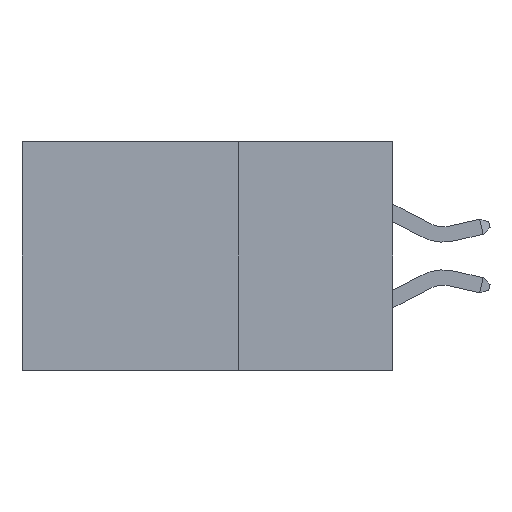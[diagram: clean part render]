
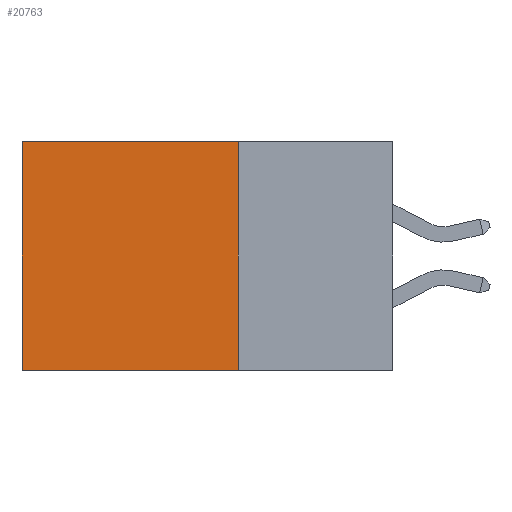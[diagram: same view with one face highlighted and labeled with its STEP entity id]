
A CAD part, left-side view. The second image highlights one B-rep face of the part: STEP entity #20763.
In plain terms, the highlighted planar face has unit normal (-1, 0, 0).
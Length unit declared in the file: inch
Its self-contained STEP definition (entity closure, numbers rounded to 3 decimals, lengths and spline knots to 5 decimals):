
#426 = ORIENTED_EDGE ( 'NONE', *, *, #22774, .F. ) ;
#922 = VERTEX_POINT ( 'NONE', #23130 ) ;
#1095 = VECTOR ( 'NONE', #3715, 39.37008 ) ;
#1285 = VERTEX_POINT ( 'NONE', #10733 ) ;
#1451 = CARTESIAN_POINT ( 'NONE',  ( 0.2875, 0.25, 0. ) ) ;
#2188 = LINE ( 'NONE', #1451, #15929 ) ;
#3715 = DIRECTION ( 'NONE',  ( 0., 0., -1. ) ) ;
#4207 = DIRECTION ( 'NONE',  ( 0., 1., 0. ) ) ;
#5421 = FACE_OUTER_BOUND ( 'NONE', #21174, .T. ) ;
#6524 = LINE ( 'NONE', #10016, #12983 ) ;
#6859 = VERTEX_POINT ( 'NONE', #26353 ) ;
#7999 = AXIS2_PLACEMENT_3D ( 'NONE', #14714, #33502, #17444 ) ;
#10016 = CARTESIAN_POINT ( 'NONE',  ( 0.2875, 0.25, -0.37 ) ) ;
#10733 = CARTESIAN_POINT ( 'NONE',  ( 0.2875, 0.6, -0.37 ) ) ;
#12983 = VECTOR ( 'NONE', #23531, 39.37008 ) ;
#14714 = CARTESIAN_POINT ( 'NONE',  ( 0.2875, 0.25, 0. ) ) ;
#15024 = EDGE_CURVE ( 'NONE', #6859, #922, #34993, .T. ) ;
#15929 = VECTOR ( 'NONE', #4207, 39.37008 ) ;
#16558 = LINE ( 'NONE', #30798, #1095 ) ;
#17122 = VERTEX_POINT ( 'NONE', #29654 ) ;
#17137 = ORIENTED_EDGE ( 'NONE', *, *, #27970, .T. ) ;
#17444 = DIRECTION ( 'NONE',  ( 0., 0., -1. ) ) ;
#19570 = ORIENTED_EDGE ( 'NONE', *, *, #25961, .T. ) ;
#20763 = ADVANCED_FACE ( 'NONE', ( #5421 ), #22733, .F. ) ;
#21174 = EDGE_LOOP ( 'NONE', ( #19570, #426, #25136, #17137 ) ) ;
#22733 = PLANE ( 'NONE',  #7999 ) ;
#22774 = EDGE_CURVE ( 'NONE', #922, #1285, #6524, .T. ) ;
#23130 = CARTESIAN_POINT ( 'NONE',  ( 0.2875, 0.25, -0.37 ) ) ;
#23531 = DIRECTION ( 'NONE',  ( 0., 1., 0. ) ) ;
#25136 = ORIENTED_EDGE ( 'NONE', *, *, #15024, .F. ) ;
#25961 = EDGE_CURVE ( 'NONE', #17122, #1285, #16558, .T. ) ;
#26353 = CARTESIAN_POINT ( 'NONE',  ( 0.2875, 0.25, 0. ) ) ;
#27045 = VECTOR ( 'NONE', #32776, 39.37008 ) ;
#27970 = EDGE_CURVE ( 'NONE', #6859, #17122, #2188, .T. ) ;
#29654 = CARTESIAN_POINT ( 'NONE',  ( 0.2875, 0.6, 0. ) ) ;
#30108 = CARTESIAN_POINT ( 'NONE',  ( 0.2875, 0.25, 0. ) ) ;
#30798 = CARTESIAN_POINT ( 'NONE',  ( 0.2875, 0.6, 0. ) ) ;
#32776 = DIRECTION ( 'NONE',  ( 0., 0., -1. ) ) ;
#33502 = DIRECTION ( 'NONE',  ( 1., 0., 0. ) ) ;
#34993 = LINE ( 'NONE', #30108, #27045 ) ;
